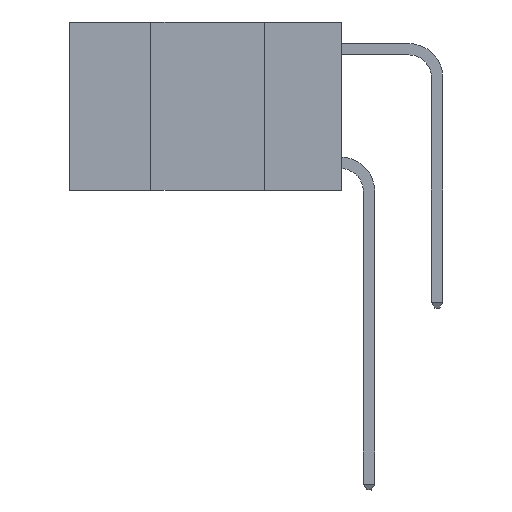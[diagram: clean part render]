
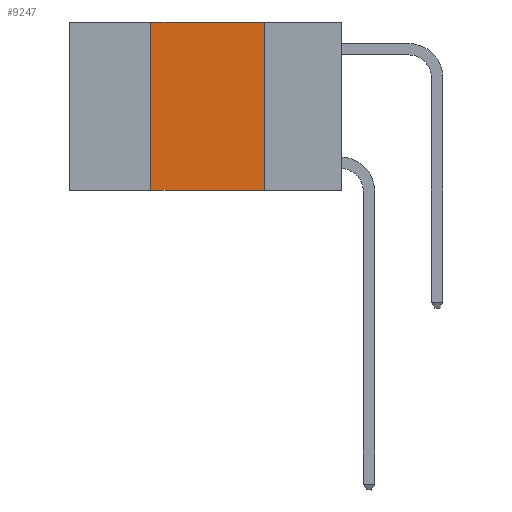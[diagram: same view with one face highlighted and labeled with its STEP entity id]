
A CAD part, left-side view. The second image highlights one B-rep face of the part: STEP entity #9247.
In plain terms, the highlighted planar face has unit normal (-1, 0, 0).
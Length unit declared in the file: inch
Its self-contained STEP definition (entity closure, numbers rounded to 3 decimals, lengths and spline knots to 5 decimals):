
#2115 = VERTEX_POINT ( 'NONE', #23616 ) ;
#3064 = LINE ( 'NONE', #11013, #22431 ) ;
#6498 = CARTESIAN_POINT ( 'NONE',  ( 0., 0.6, 0. ) ) ;
#6906 = LINE ( 'NONE', #22563, #19507 ) ;
#7193 = AXIS2_PLACEMENT_3D ( 'NONE', #6498, #8713, #8186 ) ;
#7242 = DIRECTION ( 'NONE',  ( 0., -1., 0. ) ) ;
#7267 = CARTESIAN_POINT ( 'NONE',  ( 0., 0.17, -0.37 ) ) ;
#8186 = DIRECTION ( 'NONE',  ( 0., 0., -1. ) ) ;
#8269 = ORIENTED_EDGE ( 'NONE', *, *, #16021, .T. ) ;
#8713 = DIRECTION ( 'NONE',  ( 1., 0., 0. ) ) ;
#9247 = ADVANCED_FACE ( 'NONE', ( #18286 ), #20488, .F. ) ;
#9832 = DIRECTION ( 'NONE',  ( 0., 0., 1. ) ) ;
#10274 = VECTOR ( 'NONE', #9832, 39.37008 ) ;
#10376 = ORIENTED_EDGE ( 'NONE', *, *, #23446, .F. ) ;
#10915 = DIRECTION ( 'NONE',  ( 0., 0., -1. ) ) ;
#10990 = VERTEX_POINT ( 'NONE', #7267 ) ;
#11013 = CARTESIAN_POINT ( 'NONE',  ( 0., 0.6, -0.37 ) ) ;
#11115 = CARTESIAN_POINT ( 'NONE',  ( 0., 0.17, 0. ) ) ;
#11542 = CARTESIAN_POINT ( 'NONE',  ( 0., 0.42, 0. ) ) ;
#13394 = VERTEX_POINT ( 'NONE', #11115 ) ;
#13603 = LINE ( 'NONE', #21338, #10274 ) ;
#14280 = ORIENTED_EDGE ( 'NONE', *, *, #16701, .F. ) ;
#14600 = LINE ( 'NONE', #16811, #20965 ) ;
#16021 = EDGE_CURVE ( 'NONE', #2115, #10990, #3064, .T. ) ;
#16701 = EDGE_CURVE ( 'NONE', #13394, #10990, #6906, .T. ) ;
#16811 = CARTESIAN_POINT ( 'NONE',  ( 0., 0.6, 0. ) ) ;
#18286 = FACE_OUTER_BOUND ( 'NONE', #25090, .T. ) ;
#19328 = ORIENTED_EDGE ( 'NONE', *, *, #25110, .F. ) ;
#19507 = VECTOR ( 'NONE', #10915, 39.37008 ) ;
#20285 = VERTEX_POINT ( 'NONE', #11542 ) ;
#20488 = PLANE ( 'NONE',  #7193 ) ;
#20965 = VECTOR ( 'NONE', #21875, 39.37008 ) ;
#21338 = CARTESIAN_POINT ( 'NONE',  ( 0., 0.42, 0. ) ) ;
#21875 = DIRECTION ( 'NONE',  ( 0., -1., 0. ) ) ;
#22431 = VECTOR ( 'NONE', #7242, 39.37008 ) ;
#22563 = CARTESIAN_POINT ( 'NONE',  ( 0., 0.17, 0. ) ) ;
#23446 = EDGE_CURVE ( 'NONE', #20285, #13394, #14600, .T. ) ;
#23616 = CARTESIAN_POINT ( 'NONE',  ( 0., 0.42, -0.37 ) ) ;
#25090 = EDGE_LOOP ( 'NONE', ( #14280, #10376, #19328, #8269 ) ) ;
#25110 = EDGE_CURVE ( 'NONE', #2115, #20285, #13603, .T. ) ;
